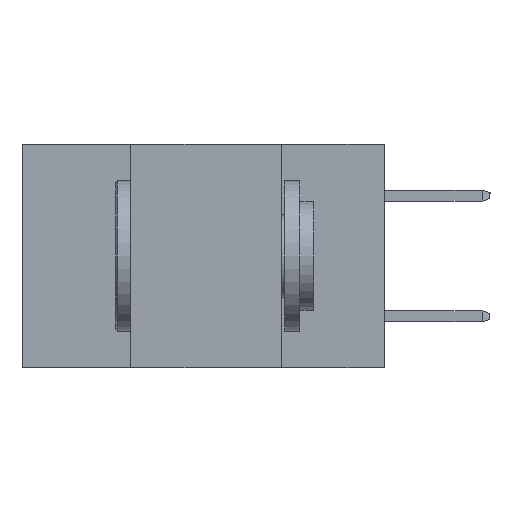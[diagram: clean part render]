
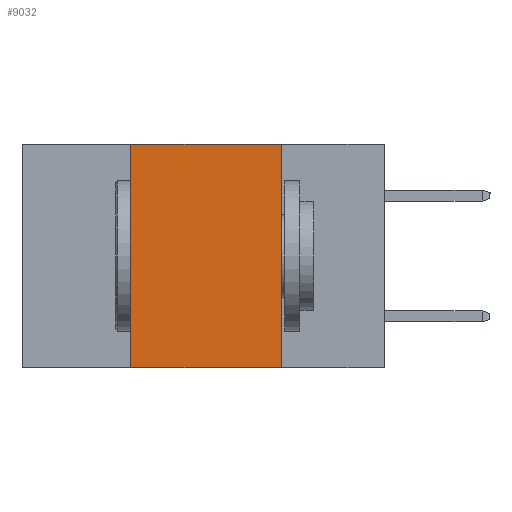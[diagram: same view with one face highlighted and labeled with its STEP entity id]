
A CAD part, left-side view. The second image highlights one B-rep face of the part: STEP entity #9032.
In plain terms, the highlighted planar face has unit normal (-1, 0, 0).
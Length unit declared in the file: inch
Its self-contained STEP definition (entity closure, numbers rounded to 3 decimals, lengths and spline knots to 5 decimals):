
#344 = EDGE_CURVE ( 'NONE', #13757, #4914, #24177, .T. ) ;
#2813 = LINE ( 'NONE', #18828, #14760 ) ;
#3458 = ORIENTED_EDGE ( 'NONE', *, *, #344, .F. ) ;
#4528 = EDGE_LOOP ( 'NONE', ( #3458, #24082, #25008, #17402 ) ) ;
#4914 = VERTEX_POINT ( 'NONE', #7693 ) ;
#5371 = EDGE_CURVE ( 'NONE', #16054, #18573, #15591, .T. ) ;
#7693 = CARTESIAN_POINT ( 'NONE',  ( 0., 0.17, -0.37 ) ) ;
#8412 = EDGE_CURVE ( 'NONE', #18573, #13757, #8443, .T. ) ;
#8443 = LINE ( 'NONE', #14322, #23904 ) ;
#9032 = ADVANCED_FACE ( 'NONE', ( #20549 ), #20806, .F. ) ;
#9838 = CARTESIAN_POINT ( 'NONE',  ( 0., 0.17, 0. ) ) ;
#9966 = CARTESIAN_POINT ( 'NONE',  ( 0., 0.42, -0.37 ) ) ;
#10654 = DIRECTION ( 'NONE',  ( 0., -1., 0. ) ) ;
#10871 = AXIS2_PLACEMENT_3D ( 'NONE', #15052, #12640, #18394 ) ;
#11417 = EDGE_CURVE ( 'NONE', #16054, #4914, #2813, .T. ) ;
#12640 = DIRECTION ( 'NONE',  ( 1., 0., 0. ) ) ;
#13757 = VERTEX_POINT ( 'NONE', #9838 ) ;
#14322 = CARTESIAN_POINT ( 'NONE',  ( 0., 0.6, 0. ) ) ;
#14760 = VECTOR ( 'NONE', #10654, 39.37008 ) ;
#15052 = CARTESIAN_POINT ( 'NONE',  ( 0., 0.6, 0. ) ) ;
#15354 = DIRECTION ( 'NONE',  ( 0., 0., 1. ) ) ;
#15591 = LINE ( 'NONE', #9966, #16507 ) ;
#16054 = VERTEX_POINT ( 'NONE', #24900 ) ;
#16244 = DIRECTION ( 'NONE',  ( 0., -1., 0. ) ) ;
#16249 = DIRECTION ( 'NONE',  ( 0., 0., -1. ) ) ;
#16366 = CARTESIAN_POINT ( 'NONE',  ( 0., 0.17, -0.37 ) ) ;
#16507 = VECTOR ( 'NONE', #15354, 39.37008 ) ;
#17105 = VECTOR ( 'NONE', #16249, 39.37008 ) ;
#17402 = ORIENTED_EDGE ( 'NONE', *, *, #11417, .T. ) ;
#18394 = DIRECTION ( 'NONE',  ( 0., 0., -1. ) ) ;
#18573 = VERTEX_POINT ( 'NONE', #19881 ) ;
#18828 = CARTESIAN_POINT ( 'NONE',  ( 0., 0.6, -0.37 ) ) ;
#19881 = CARTESIAN_POINT ( 'NONE',  ( 0., 0.42, 0. ) ) ;
#20549 = FACE_OUTER_BOUND ( 'NONE', #4528, .T. ) ;
#20806 = PLANE ( 'NONE',  #10871 ) ;
#23904 = VECTOR ( 'NONE', #16244, 39.37008 ) ;
#24082 = ORIENTED_EDGE ( 'NONE', *, *, #8412, .F. ) ;
#24177 = LINE ( 'NONE', #16366, #17105 ) ;
#24900 = CARTESIAN_POINT ( 'NONE',  ( 0., 0.42, -0.37 ) ) ;
#25008 = ORIENTED_EDGE ( 'NONE', *, *, #5371, .F. ) ;
